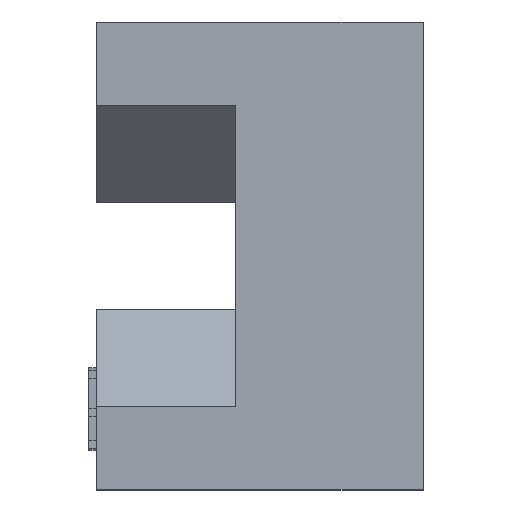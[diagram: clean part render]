
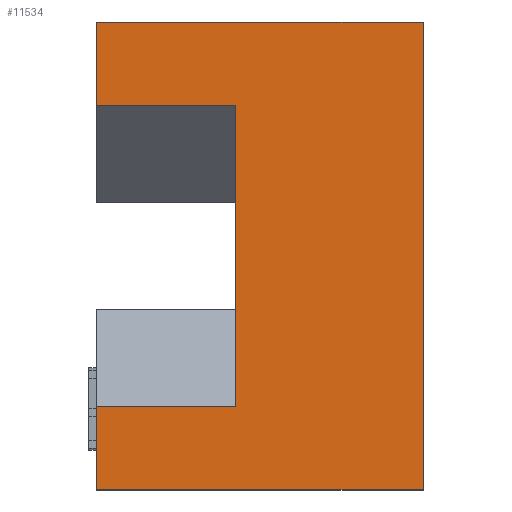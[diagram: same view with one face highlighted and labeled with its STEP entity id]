
A CAD part, left-side view. The second image highlights one B-rep face of the part: STEP entity #11534.
In plain terms, the highlighted planar face has unit normal (-1, 0, 0).
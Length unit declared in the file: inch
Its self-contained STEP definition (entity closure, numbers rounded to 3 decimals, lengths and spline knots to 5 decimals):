
#223 = DIRECTION ( 'NONE',  ( 0., -1., 0. ) ) ;
#481 = CARTESIAN_POINT ( 'NONE',  ( -3.1875, 0.218, -0.156 ) ) ;
#482 = CARTESIAN_POINT ( 'NONE',  ( -3.1875, 0.218, -0.156 ) ) ;
#526 = DIRECTION ( 'NONE',  ( 0., 0., -1. ) ) ;
#665 = VECTOR ( 'NONE', #11346, 39.37008 ) ;
#678 = ORIENTED_EDGE ( 'NONE', *, *, #8904, .T. ) ;
#754 = VERTEX_POINT ( 'NONE', #7399 ) ;
#897 = VERTEX_POINT ( 'NONE', #8366 ) ;
#954 = ORIENTED_EDGE ( 'NONE', *, *, #13997, .T. ) ;
#1105 = CARTESIAN_POINT ( 'NONE',  ( -3.1875, 0.218, 0.156 ) ) ;
#1140 = VERTEX_POINT ( 'NONE', #13608 ) ;
#1239 = ORIENTED_EDGE ( 'NONE', *, *, #10027, .T. ) ;
#1329 = EDGE_LOOP ( 'NONE', ( #11150, #678, #9289, #954, #1239, #12295, #13817, #9224 ) ) ;
#1404 = PLANE ( 'NONE',  #11748 ) ;
#1657 = VECTOR ( 'NONE', #7866, 39.37008 ) ;
#2487 = VERTEX_POINT ( 'NONE', #6184 ) ;
#2693 = VERTEX_POINT ( 'NONE', #481 ) ;
#3017 = EDGE_CURVE ( 'NONE', #2693, #897, #12101, .T. ) ;
#3754 = CARTESIAN_POINT ( 'NONE',  ( -3.1875, 0., -0.156 ) ) ;
#3755 = FACE_OUTER_BOUND ( 'NONE', #1329, .T. ) ;
#4387 = LINE ( 'NONE', #10075, #5924 ) ;
#4403 = VECTOR ( 'NONE', #9264, 39.37008 ) ;
#5924 = VECTOR ( 'NONE', #223, 39.37008 ) ;
#6184 = CARTESIAN_POINT ( 'NONE',  ( -3.1875, 0.218, 0.1005 ) ) ;
#6466 = CARTESIAN_POINT ( 'NONE',  ( -3.1875, 0.125, 0.1005 ) ) ;
#6587 = VERTEX_POINT ( 'NONE', #1105 ) ;
#6705 = CARTESIAN_POINT ( 'NONE',  ( -3.1875, 0.218, -0.156 ) ) ;
#6715 = CARTESIAN_POINT ( 'NONE',  ( -3.1875, 0.218, 0.156 ) ) ;
#6910 = CARTESIAN_POINT ( 'NONE',  ( -3.1875, 0.125, -0.1005 ) ) ;
#7137 = CARTESIAN_POINT ( 'NONE',  ( -3.1875, 0.218, -0.156 ) ) ;
#7399 = CARTESIAN_POINT ( 'NONE',  ( -3.1875, 0.125, 0.1005 ) ) ;
#7412 = DIRECTION ( 'NONE',  ( 0., 1., 0. ) ) ;
#7866 = DIRECTION ( 'NONE',  ( 0., 0., 1. ) ) ;
#8366 = CARTESIAN_POINT ( 'NONE',  ( -3.1875, 0.218, -0.1005 ) ) ;
#8904 = EDGE_CURVE ( 'NONE', #13629, #897, #10716, .T. ) ;
#8948 = DIRECTION ( 'NONE',  ( 0., -1., 0. ) ) ;
#9150 = EDGE_CURVE ( 'NONE', #13629, #754, #10409, .T. ) ;
#9224 = ORIENTED_EDGE ( 'NONE', *, *, #13908, .F. ) ;
#9264 = DIRECTION ( 'NONE',  ( 0., 0., 1. ) ) ;
#9289 = ORIENTED_EDGE ( 'NONE', *, *, #3017, .F. ) ;
#9494 = CARTESIAN_POINT ( 'NONE',  ( -3.1875, 0.125, -0.1005 ) ) ;
#9664 = DIRECTION ( 'NONE',  ( 0., 0., 1. ) ) ;
#10027 = EDGE_CURVE ( 'NONE', #10993, #1140, #13980, .T. ) ;
#10075 = CARTESIAN_POINT ( 'NONE',  ( -3.1875, 0.218, -0.156 ) ) ;
#10143 = VECTOR ( 'NONE', #10425, 39.37008 ) ;
#10305 = VECTOR ( 'NONE', #7412, 39.37008 ) ;
#10358 = VECTOR ( 'NONE', #8948, 39.37008 ) ;
#10409 = LINE ( 'NONE', #13868, #4403 ) ;
#10425 = DIRECTION ( 'NONE',  ( 0., 1., 0. ) ) ;
#10716 = LINE ( 'NONE', #9494, #10143 ) ;
#10993 = VERTEX_POINT ( 'NONE', #3754 ) ;
#11150 = ORIENTED_EDGE ( 'NONE', *, *, #9150, .F. ) ;
#11183 = VECTOR ( 'NONE', #9664, 39.37008 ) ;
#11346 = DIRECTION ( 'NONE',  ( 0., 0., 1. ) ) ;
#11534 = ADVANCED_FACE ( 'NONE', ( #3755 ), #1404, .F. ) ;
#11748 = AXIS2_PLACEMENT_3D ( 'NONE', #7137, #13481, #526 ) ;
#11820 = EDGE_CURVE ( 'NONE', #6587, #1140, #12186, .T. ) ;
#11827 = CARTESIAN_POINT ( 'NONE',  ( -3.1875, 0., -0.156 ) ) ;
#12101 = LINE ( 'NONE', #6705, #1657 ) ;
#12186 = LINE ( 'NONE', #6715, #10358 ) ;
#12295 = ORIENTED_EDGE ( 'NONE', *, *, #11820, .F. ) ;
#12489 = LINE ( 'NONE', #482, #665 ) ;
#12945 = LINE ( 'NONE', #6466, #10305 ) ;
#13124 = EDGE_CURVE ( 'NONE', #2487, #6587, #12489, .T. ) ;
#13481 = DIRECTION ( 'NONE',  ( 1., 0., 0. ) ) ;
#13608 = CARTESIAN_POINT ( 'NONE',  ( -3.1875, 0., 0.156 ) ) ;
#13629 = VERTEX_POINT ( 'NONE', #6910 ) ;
#13817 = ORIENTED_EDGE ( 'NONE', *, *, #13124, .F. ) ;
#13868 = CARTESIAN_POINT ( 'NONE',  ( -3.1875, 0.125, -0.1005 ) ) ;
#13908 = EDGE_CURVE ( 'NONE', #754, #2487, #12945, .T. ) ;
#13980 = LINE ( 'NONE', #11827, #11183 ) ;
#13997 = EDGE_CURVE ( 'NONE', #2693, #10993, #4387, .T. ) ;
